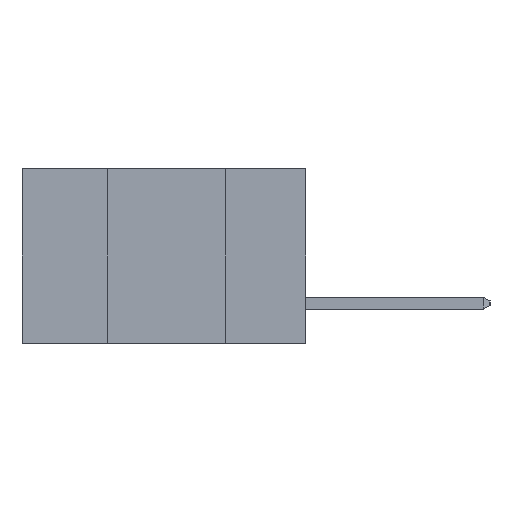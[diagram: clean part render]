
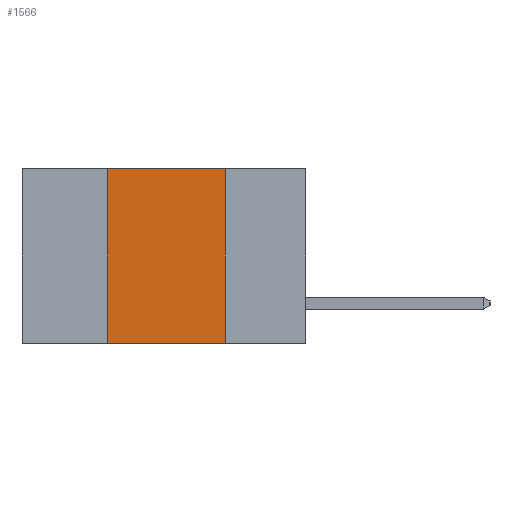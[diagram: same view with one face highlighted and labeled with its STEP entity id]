
A CAD part, left-side view. The second image highlights one B-rep face of the part: STEP entity #1566.
In plain terms, the highlighted planar face has unit normal (-1, 0, 0).
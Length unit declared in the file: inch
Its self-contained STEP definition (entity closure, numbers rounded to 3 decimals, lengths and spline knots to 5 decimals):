
#398 = EDGE_CURVE ( 'NONE', #6478, #9421, #915, .T. ) ;
#915 = LINE ( 'NONE', #11855, #11339 ) ;
#1435 = ORIENTED_EDGE ( 'NONE', *, *, #8718, .F. ) ;
#1566 = ADVANCED_FACE ( 'NONE', ( #7934 ), #11202, .F. ) ;
#1636 = AXIS2_PLACEMENT_3D ( 'NONE', #2590, #5199, #16218 ) ;
#2016 = DIRECTION ( 'NONE',  ( 0., -1., 0. ) ) ;
#2133 = VECTOR ( 'NONE', #7183, 39.37008 ) ;
#2590 = CARTESIAN_POINT ( 'NONE',  ( 0., 0.6, 0. ) ) ;
#3204 = ORIENTED_EDGE ( 'NONE', *, *, #398, .F. ) ;
#3224 = EDGE_LOOP ( 'NONE', ( #1435, #3204, #3867, #11850 ) ) ;
#3445 = CARTESIAN_POINT ( 'NONE',  ( 0., 0.17, -0.37 ) ) ;
#3624 = VECTOR ( 'NONE', #5504, 39.37008 ) ;
#3867 = ORIENTED_EDGE ( 'NONE', *, *, #7811, .F. ) ;
#4110 = CARTESIAN_POINT ( 'NONE',  ( 0., 0.6, -0.37 ) ) ;
#4938 = CARTESIAN_POINT ( 'NONE',  ( 0., 0.42, 0. ) ) ;
#5187 = VERTEX_POINT ( 'NONE', #3445 ) ;
#5199 = DIRECTION ( 'NONE',  ( 1., 0., 0. ) ) ;
#5504 = DIRECTION ( 'NONE',  ( 0., -1., 0. ) ) ;
#6001 = VERTEX_POINT ( 'NONE', #10758 ) ;
#6040 = EDGE_CURVE ( 'NONE', #6001, #5187, #7305, .T. ) ;
#6140 = LINE ( 'NONE', #16738, #15706 ) ;
#6302 = LINE ( 'NONE', #11175, #2133 ) ;
#6478 = VERTEX_POINT ( 'NONE', #4938 ) ;
#7183 = DIRECTION ( 'NONE',  ( 0., 0., -1. ) ) ;
#7305 = LINE ( 'NONE', #4110, #3624 ) ;
#7811 = EDGE_CURVE ( 'NONE', #6001, #6478, #6140, .T. ) ;
#7934 = FACE_OUTER_BOUND ( 'NONE', #3224, .T. ) ;
#8718 = EDGE_CURVE ( 'NONE', #9421, #5187, #6302, .T. ) ;
#9073 = DIRECTION ( 'NONE',  ( 0., 0., 1. ) ) ;
#9421 = VERTEX_POINT ( 'NONE', #9845 ) ;
#9845 = CARTESIAN_POINT ( 'NONE',  ( 0., 0.17, 0. ) ) ;
#10758 = CARTESIAN_POINT ( 'NONE',  ( 0., 0.42, -0.37 ) ) ;
#11175 = CARTESIAN_POINT ( 'NONE',  ( 0., 0.17, 0. ) ) ;
#11202 = PLANE ( 'NONE',  #1636 ) ;
#11339 = VECTOR ( 'NONE', #2016, 39.37008 ) ;
#11850 = ORIENTED_EDGE ( 'NONE', *, *, #6040, .T. ) ;
#11855 = CARTESIAN_POINT ( 'NONE',  ( 0., 0.6, 0. ) ) ;
#15706 = VECTOR ( 'NONE', #9073, 39.37008 ) ;
#16218 = DIRECTION ( 'NONE',  ( 0., 0., -1. ) ) ;
#16738 = CARTESIAN_POINT ( 'NONE',  ( 0., 0.42, 0. ) ) ;
